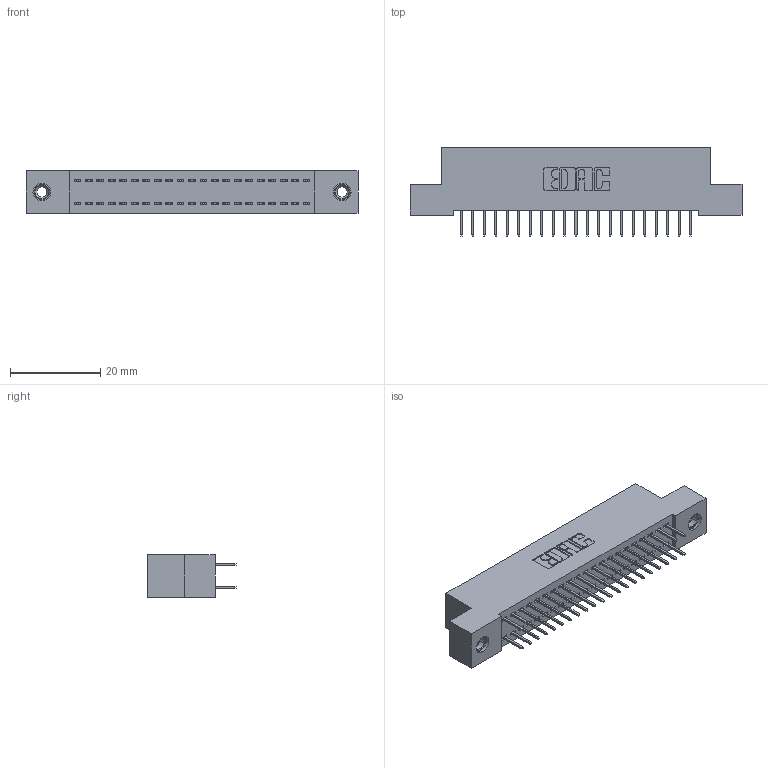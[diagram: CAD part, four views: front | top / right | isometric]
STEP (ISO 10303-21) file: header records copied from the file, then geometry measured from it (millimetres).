
FILE_DESCRIPTION (( 'STEP AP203' ), '1' );
FILE_NAME ('342-042-524-208.STEP', '2018-08-12T02:43:34', ( '' ), ( '' ), 'SwSTEP 2.0', 'SolidWorks 2016', '' );
FILE_SCHEMA (( 'CONFIG_CONTROL_DESIGN' ));
Length unit declared in the file: inch
Products named in the file (4): 342 Part_TI; 345-292-001_345-293-124; 345-250-001_345-250-003-102; 342-042-524-208
Assembly tree (45 placements, depth 2):
  342-042-524-208
    342 Part_TI
    345-292-001_345-293-124  x42
    345-250-001_345-250-003-102  x2
Bounding box: 73.66 x 19.69 x 9.4 mm (x, y, z)
Volume: 6449.7 mm3; surface area: 9826 mm2
Topology: 45 solids, 45 shells, 2522 faces, 7113 edges, 4566 vertices
Faces by surface type: plane 1862, cylinder 644, cone 12, torus 4
Entity records: 17354 total; most frequent: CARTESIAN_POINT 2881, ORIENTED_EDGE 2810, DIRECTION 2531, EDGE_CURVE 1405, LINE 1261, VECTOR 1261, VERTEX_POINT 928, AXIS2_PLACEMENT_3D 635
